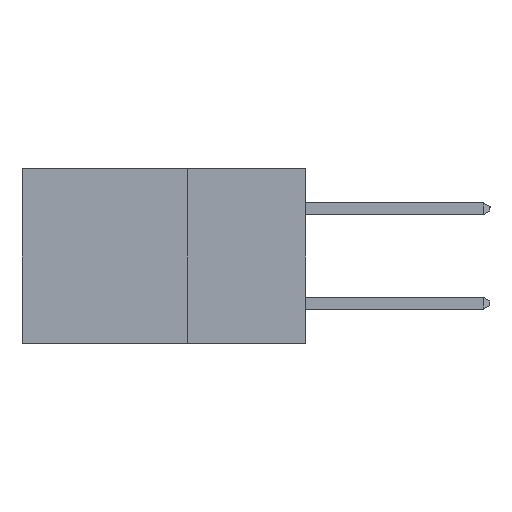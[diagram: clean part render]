
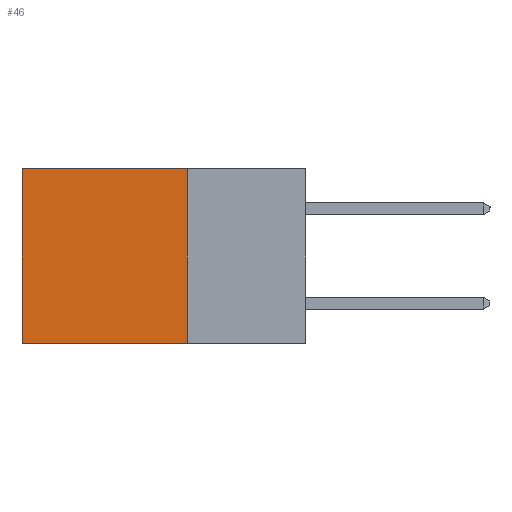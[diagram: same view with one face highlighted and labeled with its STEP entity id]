
A CAD part, left-side view. The second image highlights one B-rep face of the part: STEP entity #46.
In plain terms, the highlighted planar face has unit normal (-1, 0, 0).
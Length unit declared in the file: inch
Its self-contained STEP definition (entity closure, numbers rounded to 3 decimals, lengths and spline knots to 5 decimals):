
#46 = ADVANCED_FACE ( 'NONE', ( #6532 ), #1730, .F. ) ;
#523 = CARTESIAN_POINT ( 'NONE',  ( 0.2615, 0.25, -0.37 ) ) ;
#639 = VERTEX_POINT ( 'NONE', #5580 ) ;
#654 = CARTESIAN_POINT ( 'NONE',  ( 0.2615, 0.25, -0.37 ) ) ;
#710 = DIRECTION ( 'NONE',  ( 1., 0., 0. ) ) ;
#717 = CARTESIAN_POINT ( 'NONE',  ( 0.2615, 0.6, -0.37 ) ) ;
#784 = VECTOR ( 'NONE', #7111, 39.37008 ) ;
#1036 = EDGE_LOOP ( 'NONE', ( #5193, #8054, #6717, #11046 ) ) ;
#1289 = LINE ( 'NONE', #4216, #784 ) ;
#1696 = EDGE_CURVE ( 'NONE', #2749, #639, #1289, .T. ) ;
#1730 = PLANE ( 'NONE',  #6254 ) ;
#1834 = EDGE_CURVE ( 'NONE', #2749, #12292, #8347, .T. ) ;
#1994 = EDGE_CURVE ( 'NONE', #12292, #8045, #2945, .T. ) ;
#2056 = DIRECTION ( 'NONE',  ( 0., 0., -1. ) ) ;
#2290 = CARTESIAN_POINT ( 'NONE',  ( 0.2615, 0.25, -0.37 ) ) ;
#2749 = VERTEX_POINT ( 'NONE', #7212 ) ;
#2945 = LINE ( 'NONE', #6849, #5671 ) ;
#4216 = CARTESIAN_POINT ( 'NONE',  ( 0.2615, 0.25, 0. ) ) ;
#4424 = DIRECTION ( 'NONE',  ( 0., 0., -1. ) ) ;
#5193 = ORIENTED_EDGE ( 'NONE', *, *, #8172, .T. ) ;
#5580 = CARTESIAN_POINT ( 'NONE',  ( 0.2615, 0.6, 0. ) ) ;
#5671 = VECTOR ( 'NONE', #11634, 39.37008 ) ;
#6254 = AXIS2_PLACEMENT_3D ( 'NONE', #654, #710, #8473 ) ;
#6532 = FACE_OUTER_BOUND ( 'NONE', #1036, .T. ) ;
#6717 = ORIENTED_EDGE ( 'NONE', *, *, #1834, .F. ) ;
#6849 = CARTESIAN_POINT ( 'NONE',  ( 0.2615, 0.25, -0.37 ) ) ;
#7111 = DIRECTION ( 'NONE',  ( 0., 1., 0. ) ) ;
#7212 = CARTESIAN_POINT ( 'NONE',  ( 0.2615, 0.25, 0. ) ) ;
#7808 = LINE ( 'NONE', #8985, #12406 ) ;
#8045 = VERTEX_POINT ( 'NONE', #717 ) ;
#8054 = ORIENTED_EDGE ( 'NONE', *, *, #1994, .F. ) ;
#8172 = EDGE_CURVE ( 'NONE', #639, #8045, #7808, .T. ) ;
#8347 = LINE ( 'NONE', #523, #10459 ) ;
#8473 = DIRECTION ( 'NONE',  ( 0., 0., -1. ) ) ;
#8985 = CARTESIAN_POINT ( 'NONE',  ( 0.2615, 0.6, -0.37 ) ) ;
#10459 = VECTOR ( 'NONE', #4424, 39.37008 ) ;
#11046 = ORIENTED_EDGE ( 'NONE', *, *, #1696, .T. ) ;
#11634 = DIRECTION ( 'NONE',  ( 0., 1., 0. ) ) ;
#12292 = VERTEX_POINT ( 'NONE', #2290 ) ;
#12406 = VECTOR ( 'NONE', #2056, 39.37008 ) ;
